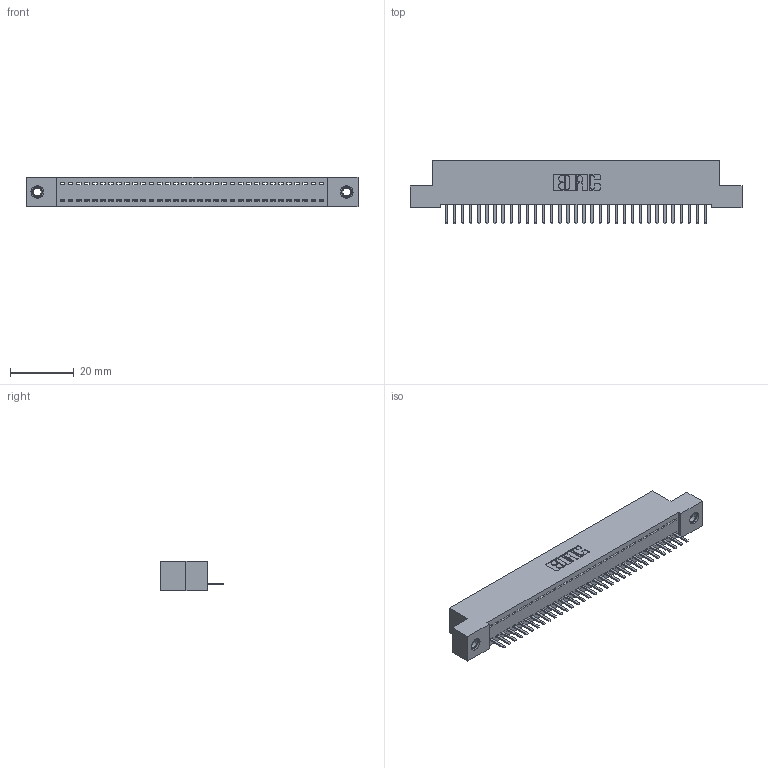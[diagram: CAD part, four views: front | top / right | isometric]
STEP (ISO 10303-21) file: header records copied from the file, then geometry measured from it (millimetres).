
FILE_DESCRIPTION (( 'STEP AP203' ), '1' );
FILE_NAME ('392-033-520-107.STEP', '2019-10-07T15:08:32', ( '' ), ( '' ), 'SwSTEP 2.0', 'SolidWorks 2016', '' );
FILE_SCHEMA (( 'CONFIG_CONTROL_DESIGN' ));
Length unit declared in the file: inch
Products named in the file (4): 342 Part_TI; 345-292-001_345-293-120; 345-250-001_345-250-005-103; 392-033-520-107
Assembly tree (36 placements, depth 2):
  392-033-520-107
    342 Part_TI
    345-292-001_345-293-120  x33
    345-250-001_345-250-005-103  x2
Bounding box: 104.14 x 20.02 x 9.4 mm (x, y, z)
Volume: 8990.2 mm3; surface area: 12762.3 mm2
Topology: 36 solids, 36 shells, 2216 faces, 6507 edges, 4242 vertices
Faces by surface type: plane 1550, cylinder 650, cone 12, torus 4
Entity records: 22506 total; most frequent: CARTESIAN_POINT 3876, ORIENTED_EDGE 3826, DIRECTION 3309, EDGE_CURVE 1913, LINE 1761, VECTOR 1761, VERTEX_POINT 1268, AXIS2_PLACEMENT_3D 774
